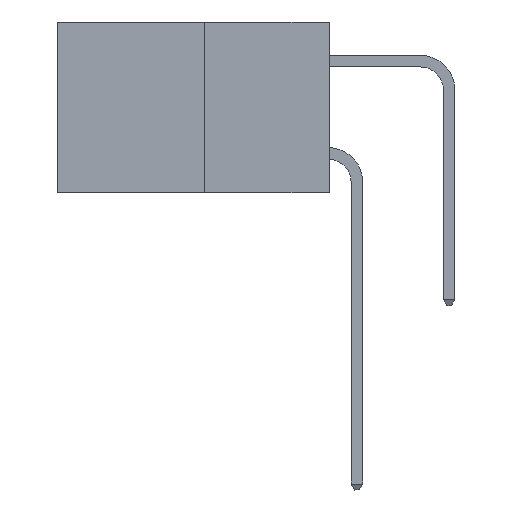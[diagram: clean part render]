
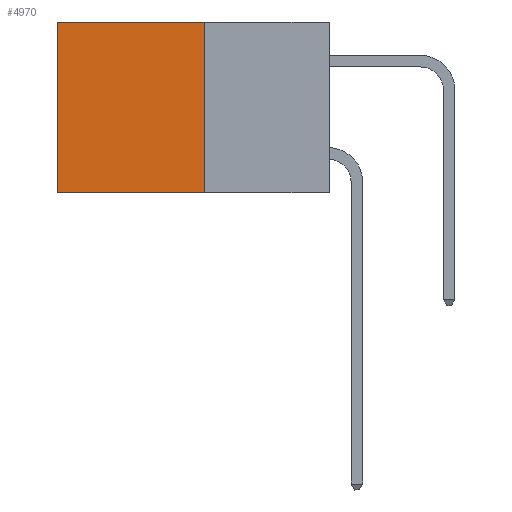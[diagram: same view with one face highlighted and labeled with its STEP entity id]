
A CAD part, left-side view. The second image highlights one B-rep face of the part: STEP entity #4970.
In plain terms, the highlighted planar face has unit normal (-1, 0, 0).
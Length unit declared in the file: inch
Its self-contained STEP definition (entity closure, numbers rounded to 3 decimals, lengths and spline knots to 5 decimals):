
#1392 = VECTOR ( 'NONE', #13621, 39.37008 ) ;
#1624 = CARTESIAN_POINT ( 'NONE',  ( 0.277, 0.27, -0.37 ) ) ;
#1717 = DIRECTION ( 'NONE',  ( 0., 0., -1. ) ) ;
#1935 = CARTESIAN_POINT ( 'NONE',  ( 0.277, 0.27, -0.37 ) ) ;
#2894 = EDGE_LOOP ( 'NONE', ( #15191, #15671, #12478, #10624 ) ) ;
#3317 = DIRECTION ( 'NONE',  ( 0., 1., 0. ) ) ;
#4538 = CARTESIAN_POINT ( 'NONE',  ( 0.277, 0.27, 0. ) ) ;
#4970 = ADVANCED_FACE ( 'NONE', ( #13315 ), #13681, .F. ) ;
#6134 = LINE ( 'NONE', #4538, #10521 ) ;
#7639 = VERTEX_POINT ( 'NONE', #1935 ) ;
#9865 = CARTESIAN_POINT ( 'NONE',  ( 0.277, 0.59, 0. ) ) ;
#10179 = CARTESIAN_POINT ( 'NONE',  ( 0.277, 0.27, -0.37 ) ) ;
#10313 = DIRECTION ( 'NONE',  ( 0., 1., 0. ) ) ;
#10364 = CARTESIAN_POINT ( 'NONE',  ( 0.277, 0.59, -0.37 ) ) ;
#10486 = LINE ( 'NONE', #1624, #18861 ) ;
#10521 = VECTOR ( 'NONE', #3317, 39.37008 ) ;
#10624 = ORIENTED_EDGE ( 'NONE', *, *, #14753, .T. ) ;
#10999 = EDGE_CURVE ( 'NONE', #15141, #15911, #14053, .T. ) ;
#11134 = LINE ( 'NONE', #10179, #19536 ) ;
#11863 = VERTEX_POINT ( 'NONE', #20898 ) ;
#12478 = ORIENTED_EDGE ( 'NONE', *, *, #15458, .F. ) ;
#13315 = FACE_OUTER_BOUND ( 'NONE', #2894, .T. ) ;
#13621 = DIRECTION ( 'NONE',  ( 0., 0., -1. ) ) ;
#13681 = PLANE ( 'NONE',  #18996 ) ;
#14053 = LINE ( 'NONE', #14593, #1392 ) ;
#14593 = CARTESIAN_POINT ( 'NONE',  ( 0.277, 0.59, -0.37 ) ) ;
#14753 = EDGE_CURVE ( 'NONE', #11863, #15141, #6134, .T. ) ;
#15075 = DIRECTION ( 'NONE',  ( 1., 0., 0. ) ) ;
#15141 = VERTEX_POINT ( 'NONE', #9865 ) ;
#15191 = ORIENTED_EDGE ( 'NONE', *, *, #10999, .T. ) ;
#15458 = EDGE_CURVE ( 'NONE', #11863, #7639, #10486, .T. ) ;
#15671 = ORIENTED_EDGE ( 'NONE', *, *, #18101, .F. ) ;
#15911 = VERTEX_POINT ( 'NONE', #10364 ) ;
#17037 = DIRECTION ( 'NONE',  ( 0., 0., -1. ) ) ;
#18101 = EDGE_CURVE ( 'NONE', #7639, #15911, #11134, .T. ) ;
#18861 = VECTOR ( 'NONE', #1717, 39.37008 ) ;
#18996 = AXIS2_PLACEMENT_3D ( 'NONE', #21050, #15075, #17037 ) ;
#19536 = VECTOR ( 'NONE', #10313, 39.37008 ) ;
#20898 = CARTESIAN_POINT ( 'NONE',  ( 0.277, 0.27, 0. ) ) ;
#21050 = CARTESIAN_POINT ( 'NONE',  ( 0.277, 0.27, -0.37 ) ) ;
